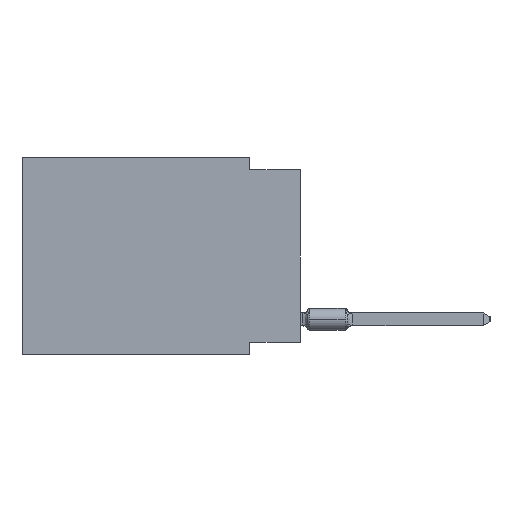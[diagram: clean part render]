
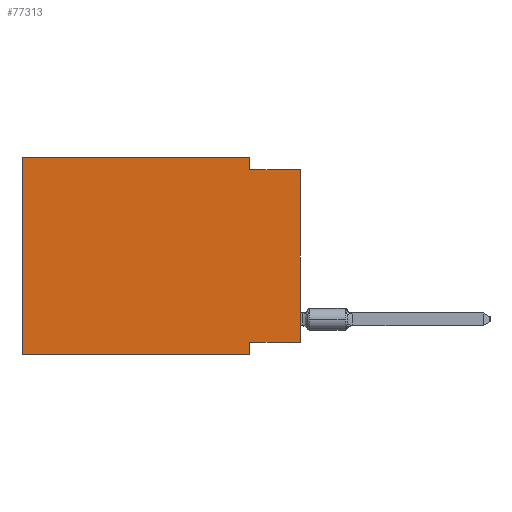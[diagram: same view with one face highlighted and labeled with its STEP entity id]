
A CAD part, left-side view. The second image highlights one B-rep face of the part: STEP entity #77313.
In plain terms, the highlighted planar face has unit normal (-1, 0, 0).
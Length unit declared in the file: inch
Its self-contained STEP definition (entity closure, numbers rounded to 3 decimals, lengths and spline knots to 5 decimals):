
#349 = VECTOR ( 'NONE', #71591, 39.37008 ) ;
#883 = VECTOR ( 'NONE', #33538, 39.37008 ) ;
#4162 = ORIENTED_EDGE ( 'NONE', *, *, #54090, .T. ) ;
#4588 = DIRECTION ( 'NONE',  ( 0., 0., -1. ) ) ;
#6483 = VECTOR ( 'NONE', #38357, 39.37008 ) ;
#8387 = EDGE_CURVE ( 'NONE', #41655, #66073, #32361, .T. ) ;
#10381 = CARTESIAN_POINT ( 'NONE',  ( 0., 0.55, 0. ) ) ;
#10571 = VERTEX_POINT ( 'NONE', #33189 ) ;
#12066 = LINE ( 'NONE', #57702, #6483 ) ;
#13383 = LINE ( 'NONE', #52851, #86441 ) ;
#14717 = CARTESIAN_POINT ( 'NONE',  ( 0., 0., -0.025 ) ) ;
#18266 = EDGE_CURVE ( 'NONE', #86214, #10571, #36231, .T. ) ;
#18506 = CARTESIAN_POINT ( 'NONE',  ( 0., 0., 0. ) ) ;
#21675 = ORIENTED_EDGE ( 'NONE', *, *, #77697, .T. ) ;
#22337 = CARTESIAN_POINT ( 'NONE',  ( 0., 0., -0.365 ) ) ;
#22484 = VERTEX_POINT ( 'NONE', #48309 ) ;
#25143 = DIRECTION ( 'NONE',  ( 0., 0., 1. ) ) ;
#27162 = CARTESIAN_POINT ( 'NONE',  ( 0., 0.1, -0.365 ) ) ;
#27399 = CARTESIAN_POINT ( 'NONE',  ( 0., 0.1, 0. ) ) ;
#28028 = LINE ( 'NONE', #22337, #71816 ) ;
#29897 = ORIENTED_EDGE ( 'NONE', *, *, #42986, .F. ) ;
#31114 = EDGE_LOOP ( 'NONE', ( #21675, #45014, #76440, #69509, #32307, #4162, #50464, #29897 ) ) ;
#31297 = CARTESIAN_POINT ( 'NONE',  ( 0., 0., -0.365 ) ) ;
#31539 = EDGE_CURVE ( 'NONE', #10571, #58068, #46709, .T. ) ;
#32307 = ORIENTED_EDGE ( 'NONE', *, *, #69022, .F. ) ;
#32361 = LINE ( 'NONE', #38518, #35182 ) ;
#33189 = CARTESIAN_POINT ( 'NONE',  ( 0., 0.1, 0. ) ) ;
#33538 = DIRECTION ( 'NONE',  ( 0., 0., -1. ) ) ;
#34559 = VERTEX_POINT ( 'NONE', #14717 ) ;
#35182 = VECTOR ( 'NONE', #58299, 39.37008 ) ;
#36231 = LINE ( 'NONE', #10381, #79336 ) ;
#38357 = DIRECTION ( 'NONE',  ( 0., -1., 0. ) ) ;
#38518 = CARTESIAN_POINT ( 'NONE',  ( 0., 0.1, -0.39 ) ) ;
#41655 = VERTEX_POINT ( 'NONE', #27162 ) ;
#42986 = EDGE_CURVE ( 'NONE', #78925, #41655, #28028, .T. ) ;
#45014 = ORIENTED_EDGE ( 'NONE', *, *, #55376, .F. ) ;
#46709 = LINE ( 'NONE', #27399, #883 ) ;
#48309 = CARTESIAN_POINT ( 'NONE',  ( 0., 0.55, -0.39 ) ) ;
#50464 = ORIENTED_EDGE ( 'NONE', *, *, #8387, .F. ) ;
#51506 = FACE_OUTER_BOUND ( 'NONE', #31114, .T. ) ;
#52571 = CARTESIAN_POINT ( 'NONE',  ( 0., 0.55, 0. ) ) ;
#52851 = CARTESIAN_POINT ( 'NONE',  ( 0., 0., -0.025 ) ) ;
#54090 = EDGE_CURVE ( 'NONE', #22484, #66073, #12066, .T. ) ;
#55376 = EDGE_CURVE ( 'NONE', #58068, #34559, #13383, .T. ) ;
#55557 = DIRECTION ( 'NONE',  ( 0., -1., 0. ) ) ;
#57677 = DIRECTION ( 'NONE',  ( 1., 0., 0. ) ) ;
#57702 = CARTESIAN_POINT ( 'NONE',  ( 0., 0.55, -0.39 ) ) ;
#58012 = LINE ( 'NONE', #18506, #349 ) ;
#58068 = VERTEX_POINT ( 'NONE', #73781 ) ;
#58299 = DIRECTION ( 'NONE',  ( 0., 0., -1. ) ) ;
#64699 = PLANE ( 'NONE',  #68988 ) ;
#66073 = VERTEX_POINT ( 'NONE', #86480 ) ;
#67593 = VECTOR ( 'NONE', #25143, 39.37008 ) ;
#68988 = AXIS2_PLACEMENT_3D ( 'NONE', #78272, #57677, #4588 ) ;
#69022 = EDGE_CURVE ( 'NONE', #22484, #86214, #76624, .T. ) ;
#69509 = ORIENTED_EDGE ( 'NONE', *, *, #18266, .F. ) ;
#71591 = DIRECTION ( 'NONE',  ( 0., 0., 1. ) ) ;
#71816 = VECTOR ( 'NONE', #76287, 39.37008 ) ;
#73781 = CARTESIAN_POINT ( 'NONE',  ( 0., 0.1, -0.025 ) ) ;
#76287 = DIRECTION ( 'NONE',  ( 0., 1., 0. ) ) ;
#76440 = ORIENTED_EDGE ( 'NONE', *, *, #31539, .F. ) ;
#76624 = LINE ( 'NONE', #85259, #67593 ) ;
#77313 = ADVANCED_FACE ( 'NONE', ( #51506 ), #64699, .F. ) ;
#77697 = EDGE_CURVE ( 'NONE', #78925, #34559, #58012, .T. ) ;
#78272 = CARTESIAN_POINT ( 'NONE',  ( 0., 0.55, 0. ) ) ;
#78925 = VERTEX_POINT ( 'NONE', #31297 ) ;
#79336 = VECTOR ( 'NONE', #55557, 39.37008 ) ;
#81356 = DIRECTION ( 'NONE',  ( 0., -1., 0. ) ) ;
#85259 = CARTESIAN_POINT ( 'NONE',  ( 0., 0.55, 0. ) ) ;
#86214 = VERTEX_POINT ( 'NONE', #52571 ) ;
#86441 = VECTOR ( 'NONE', #81356, 39.37008 ) ;
#86480 = CARTESIAN_POINT ( 'NONE',  ( 0., 0.1, -0.39 ) ) ;
